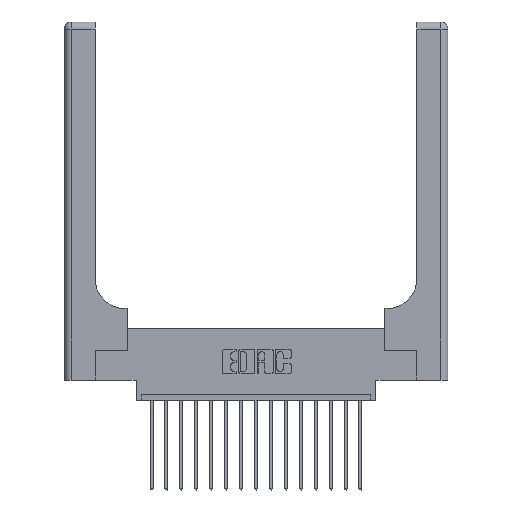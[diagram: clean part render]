
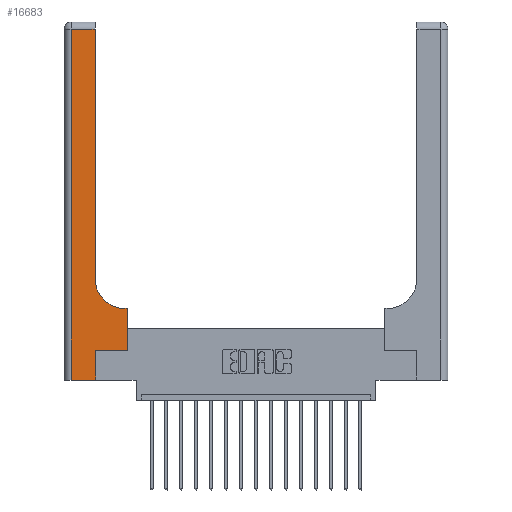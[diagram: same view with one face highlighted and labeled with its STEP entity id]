
A CAD part, top view. The second image highlights one B-rep face of the part: STEP entity #16683.
In plain terms, the highlighted planar face has unit normal (0, 0, 1).
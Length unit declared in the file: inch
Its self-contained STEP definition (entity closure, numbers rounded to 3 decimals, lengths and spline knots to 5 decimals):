
#30 = DIRECTION ( 'NONE',  ( 1., 0., 0. ) ) ;
#890 = CARTESIAN_POINT ( 'NONE',  ( 0.528, 0.25, 0.37 ) ) ;
#1104 = CARTESIAN_POINT ( 'NONE',  ( 0.26, 0.85, 0.37 ) ) ;
#1179 = VERTEX_POINT ( 'NONE', #6160 ) ;
#1258 = EDGE_CURVE ( 'NONE', #9710, #5200, #14079, .T. ) ;
#1586 = VECTOR ( 'NONE', #12091, 39.37008 ) ;
#1686 = DIRECTION ( 'NONE',  ( -1., 0., 0. ) ) ;
#1981 = CARTESIAN_POINT ( 'NONE',  ( 0.265, 0., 0.37 ) ) ;
#2131 = VECTOR ( 'NONE', #9248, 39.37008 ) ;
#2370 = VECTOR ( 'NONE', #1686, 39.37008 ) ;
#2427 = EDGE_LOOP ( 'NONE', ( #17245, #15599, #15876, #17933, #6685, #17830, #8448, #11789, #6316 ) ) ;
#2815 = DIRECTION ( 'NONE',  ( -1., 0., 0. ) ) ;
#3043 = AXIS2_PLACEMENT_3D ( 'NONE', #4247, #10016, #2815 ) ;
#3164 = VERTEX_POINT ( 'NONE', #12162 ) ;
#3178 = EDGE_CURVE ( 'NONE', #10699, #1179, #17924, .T. ) ;
#3412 = CARTESIAN_POINT ( 'NONE',  ( 0.26, 2.94, 0.37 ) ) ;
#3499 = CARTESIAN_POINT ( 'NONE',  ( 0.265, 0., 0.37 ) ) ;
#4247 = CARTESIAN_POINT ( 'NONE',  ( 0., 3., 0.37 ) ) ;
#4408 = CARTESIAN_POINT ( 'NONE',  ( 0.06, 2.94, 0.37 ) ) ;
#5172 = VERTEX_POINT ( 'NONE', #890 ) ;
#5200 = VERTEX_POINT ( 'NONE', #3412 ) ;
#5334 = LINE ( 'NONE', #16970, #18154 ) ;
#5376 = EDGE_CURVE ( 'NONE', #5200, #9885, #18386, .T. ) ;
#5674 = PLANE ( 'NONE',  #3043 ) ;
#5687 = CARTESIAN_POINT ( 'NONE',  ( 0.528, 0.6, 0.37 ) ) ;
#6160 = CARTESIAN_POINT ( 'NONE',  ( 0.51, 0.6, 0.37 ) ) ;
#6316 = ORIENTED_EDGE ( 'NONE', *, *, #9811, .T. ) ;
#6529 = VERTEX_POINT ( 'NONE', #12144 ) ;
#6685 = ORIENTED_EDGE ( 'NONE', *, *, #15405, .T. ) ;
#7083 = AXIS2_PLACEMENT_3D ( 'NONE', #18610, #11423, #15618 ) ;
#7198 = CARTESIAN_POINT ( 'NONE',  ( 0.06, 3., 0.37 ) ) ;
#7342 = EDGE_CURVE ( 'NONE', #5172, #10699, #17953, .T. ) ;
#7544 = LINE ( 'NONE', #1981, #2131 ) ;
#8448 = ORIENTED_EDGE ( 'NONE', *, *, #7342, .T. ) ;
#8643 = CARTESIAN_POINT ( 'NONE',  ( 0., 0., 0.37 ) ) ;
#8707 = LINE ( 'NONE', #7198, #9093 ) ;
#8973 = VECTOR ( 'NONE', #18578, 39.37008 ) ;
#9093 = VECTOR ( 'NONE', #12965, 39.37008 ) ;
#9228 = CARTESIAN_POINT ( 'NONE',  ( 0.26, 0.6, 0.37 ) ) ;
#9248 = DIRECTION ( 'NONE',  ( 0., 1., 0. ) ) ;
#9455 = DIRECTION ( 'NONE',  ( 0., 1., 0. ) ) ;
#9535 = VECTOR ( 'NONE', #9455, 39.37008 ) ;
#9710 = VERTEX_POINT ( 'NONE', #1104 ) ;
#9811 = EDGE_CURVE ( 'NONE', #1179, #9710, #11607, .T. ) ;
#9885 = VERTEX_POINT ( 'NONE', #4408 ) ;
#10016 = DIRECTION ( 'NONE',  ( 0., 0., -1. ) ) ;
#10324 = LINE ( 'NONE', #8643, #16704 ) ;
#10655 = EDGE_CURVE ( 'NONE', #9885, #6529, #8707, .T. ) ;
#10699 = VERTEX_POINT ( 'NONE', #5687 ) ;
#11423 = DIRECTION ( 'NONE',  ( 0., 0., -1. ) ) ;
#11607 = CIRCLE ( 'NONE', #7083, 0.25 ) ;
#11789 = ORIENTED_EDGE ( 'NONE', *, *, #3178, .T. ) ;
#11996 = EDGE_CURVE ( 'NONE', #6529, #18698, #10324, .T. ) ;
#12091 = DIRECTION ( 'NONE',  ( 0., 1., 0. ) ) ;
#12144 = CARTESIAN_POINT ( 'NONE',  ( 0.06, 0., 0.37 ) ) ;
#12162 = CARTESIAN_POINT ( 'NONE',  ( 0.265, 0.25, 0.37 ) ) ;
#12635 = DIRECTION ( 'NONE',  ( 1., 0., 0. ) ) ;
#12809 = CARTESIAN_POINT ( 'NONE',  ( 0., 2.94, 0.37 ) ) ;
#12872 = FACE_OUTER_BOUND ( 'NONE', #2427, .T. ) ;
#12965 = DIRECTION ( 'NONE',  ( 0., -1., 0. ) ) ;
#14079 = LINE ( 'NONE', #18346, #9535 ) ;
#15405 = EDGE_CURVE ( 'NONE', #18698, #3164, #7544, .T. ) ;
#15599 = ORIENTED_EDGE ( 'NONE', *, *, #5376, .T. ) ;
#15618 = DIRECTION ( 'NONE',  ( 1., 0., 0. ) ) ;
#15876 = ORIENTED_EDGE ( 'NONE', *, *, #10655, .T. ) ;
#16233 = EDGE_CURVE ( 'NONE', #3164, #5172, #5334, .T. ) ;
#16683 = ADVANCED_FACE ( 'NONE', ( #12872 ), #5674, .F. ) ;
#16704 = VECTOR ( 'NONE', #30, 39.37008 ) ;
#16970 = CARTESIAN_POINT ( 'NONE',  ( 0.265, 0.25, 0.37 ) ) ;
#17245 = ORIENTED_EDGE ( 'NONE', *, *, #1258, .T. ) ;
#17761 = CARTESIAN_POINT ( 'NONE',  ( 0.528, 0.25, 0.37 ) ) ;
#17830 = ORIENTED_EDGE ( 'NONE', *, *, #16233, .T. ) ;
#17924 = LINE ( 'NONE', #9228, #2370 ) ;
#17933 = ORIENTED_EDGE ( 'NONE', *, *, #11996, .T. ) ;
#17953 = LINE ( 'NONE', #17761, #1586 ) ;
#18154 = VECTOR ( 'NONE', #12635, 39.37008 ) ;
#18346 = CARTESIAN_POINT ( 'NONE',  ( 0.26, 3., 0.37 ) ) ;
#18386 = LINE ( 'NONE', #12809, #8973 ) ;
#18578 = DIRECTION ( 'NONE',  ( -1., 0., 0. ) ) ;
#18610 = CARTESIAN_POINT ( 'NONE',  ( 0.51, 0.85, 0.37 ) ) ;
#18698 = VERTEX_POINT ( 'NONE', #3499 ) ;
